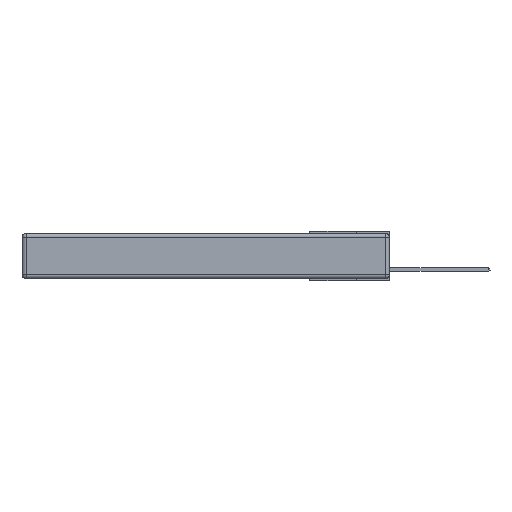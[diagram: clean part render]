
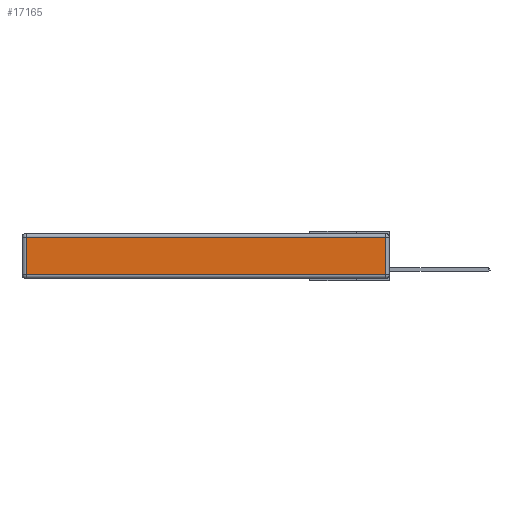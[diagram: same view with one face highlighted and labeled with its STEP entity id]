
A CAD part, left-side view. The second image highlights one B-rep face of the part: STEP entity #17165.
In plain terms, the highlighted planar face has unit normal (-1, 0, 0).
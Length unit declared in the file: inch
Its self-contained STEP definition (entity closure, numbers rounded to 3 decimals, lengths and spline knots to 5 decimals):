
#1360 = CARTESIAN_POINT ( 'NONE',  ( 0., 0.03, -0.313 ) ) ;
#2665 = CARTESIAN_POINT ( 'NONE',  ( 0., 2.72, -0.343 ) ) ;
#2981 = CARTESIAN_POINT ( 'NONE',  ( 0., 2.72, -0.313 ) ) ;
#5183 = EDGE_CURVE ( 'NONE', #18840, #12133, #8181, .T. ) ;
#7655 = AXIS2_PLACEMENT_3D ( 'NONE', #11487, #16701, #29063 ) ;
#8181 = LINE ( 'NONE', #22890, #28776 ) ;
#8676 = VECTOR ( 'NONE', #16169, 39.37008 ) ;
#9081 = FACE_OUTER_BOUND ( 'NONE', #15271, .T. ) ;
#10041 = VERTEX_POINT ( 'NONE', #1360 ) ;
#10999 = EDGE_CURVE ( 'NONE', #12133, #23972, #21405, .T. ) ;
#11353 = CARTESIAN_POINT ( 'NONE',  ( 0., 0.03, -0.343 ) ) ;
#11487 = CARTESIAN_POINT ( 'NONE',  ( 0., 0., -0.343 ) ) ;
#11785 = LINE ( 'NONE', #11353, #8676 ) ;
#12133 = VERTEX_POINT ( 'NONE', #28547 ) ;
#13561 = ORIENTED_EDGE ( 'NONE', *, *, #24987, .T. ) ;
#13710 = CARTESIAN_POINT ( 'NONE',  ( 0., 0.03, -0.03 ) ) ;
#15271 = EDGE_LOOP ( 'NONE', ( #13561, #18174, #24769, #26488 ) ) ;
#16169 = DIRECTION ( 'NONE',  ( 0., 0., 1. ) ) ;
#16701 = DIRECTION ( 'NONE',  ( -1., 0., 0. ) ) ;
#17165 = ADVANCED_FACE ( 'NONE', ( #9081 ), #19815, .T. ) ;
#17903 = CARTESIAN_POINT ( 'NONE',  ( 0., 0., -0.313 ) ) ;
#18174 = ORIENTED_EDGE ( 'NONE', *, *, #31295, .T. ) ;
#18840 = VERTEX_POINT ( 'NONE', #13710 ) ;
#19815 = PLANE ( 'NONE',  #7655 ) ;
#21405 = LINE ( 'NONE', #2665, #30753 ) ;
#22388 = LINE ( 'NONE', #17903, #30190 ) ;
#22890 = CARTESIAN_POINT ( 'NONE',  ( 0., 2.75, -0.03 ) ) ;
#23972 = VERTEX_POINT ( 'NONE', #2981 ) ;
#24769 = ORIENTED_EDGE ( 'NONE', *, *, #5183, .T. ) ;
#24987 = EDGE_CURVE ( 'NONE', #23972, #10041, #22388, .T. ) ;
#25236 = DIRECTION ( 'NONE',  ( 0., -1., 0. ) ) ;
#26488 = ORIENTED_EDGE ( 'NONE', *, *, #10999, .T. ) ;
#27686 = DIRECTION ( 'NONE',  ( 0., 1., 0. ) ) ;
#28547 = CARTESIAN_POINT ( 'NONE',  ( 0., 2.72, -0.03 ) ) ;
#28776 = VECTOR ( 'NONE', #27686, 39.37008 ) ;
#29063 = DIRECTION ( 'NONE',  ( 0., 0., 1. ) ) ;
#29834 = DIRECTION ( 'NONE',  ( 0., 0., -1. ) ) ;
#30190 = VECTOR ( 'NONE', #25236, 39.37008 ) ;
#30753 = VECTOR ( 'NONE', #29834, 39.37008 ) ;
#31295 = EDGE_CURVE ( 'NONE', #10041, #18840, #11785, .T. ) ;
